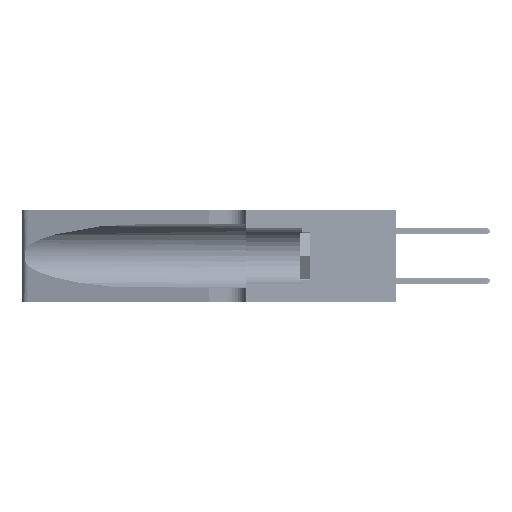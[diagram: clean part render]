
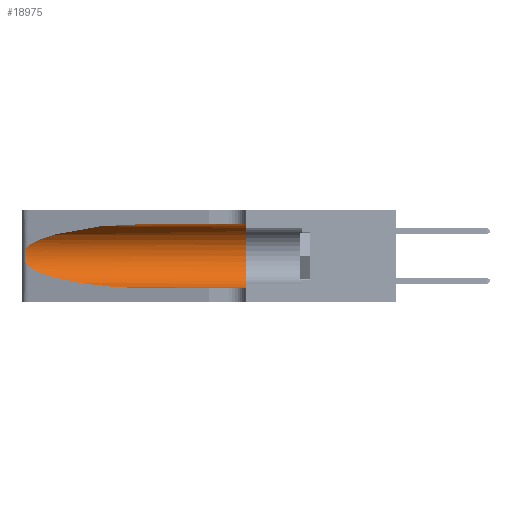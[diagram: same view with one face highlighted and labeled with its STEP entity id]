
A CAD part, left-side view. The second image highlights one B-rep face of the part: STEP entity #18975.
In plain terms, the highlighted cylindrical face has radius 3.308 mm (diameter 6.617 mm), a partial arc.
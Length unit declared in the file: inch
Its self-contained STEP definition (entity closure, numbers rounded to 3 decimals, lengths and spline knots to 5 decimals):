
#648 = EDGE_CURVE ( 'NONE', #43792, #8426, #23470, .T. ) ;
#1155 = CARTESIAN_POINT ( 'NONE',  ( 0.25487, 1.22718, 0.14631 ) ) ;
#2716 = CARTESIAN_POINT ( 'NONE',  ( 0.1305, 1.61858, 0.31525 ) ) ;
#3022 = DIRECTION ( 'NONE',  ( 0., 0., 1. ) ) ;
#4102 = CARTESIAN_POINT ( 'NONE',  ( 0.1305, 1.61858, 0.185 ) ) ;
#4693 = ORIENTED_EDGE ( 'NONE', *, *, #30047, .T. ) ;
#5092 = CARTESIAN_POINT ( 'NONE',  ( 0.25487, 1.22718, 0.14631 ) ) ;
#5726 = CARTESIAN_POINT ( 'NONE',  ( 0.26018, 1.23835, 0.19895 ) ) ;
#5967 = CIRCLE ( 'NONE', #16282, 0.13025 ) ;
#8426 = VERTEX_POINT ( 'NONE', #18879 ) ;
#8588 = CARTESIAN_POINT ( 'NONE',  ( 0.25487, 1.22718, 0.14631 ) ) ;
#9686 = CYLINDRICAL_SURFACE ( 'NONE', #45352, 0.13025 ) ;
#9708 = CARTESIAN_POINT ( 'NONE',  ( 0.1305, 0.72297, 0.31525 ) ) ;
#12324 = CARTESIAN_POINT ( 'NONE',  ( 0.1305, 0.35, 0.31525 ) ) ;
#12481 = CARTESIAN_POINT ( 'NONE',  ( 0.18966, 0.96281, 0.05475 ) ) ;
#12839 = CARTESIAN_POINT ( 'NONE',  ( 0.25639, 1.23184, 0.21858 ) ) ;
#12999 = CARTESIAN_POINT ( 'NONE',  ( 0.26017, 1.23833, 0.17102 ) ) ;
#13162 = CARTESIAN_POINT ( 'NONE',  ( 0.26075, 1.23896, 0.178 ) ) ;
#13328 = CARTESIAN_POINT ( 'NONE',  ( 0.25487, 1.22718, 0.22369 ) ) ;
#14504 = B_SPLINE_CURVE_WITH_KNOTS ( 'NONE', 3,
 ( #13328, #24491, #12839, #16703, #28889, #5726, #36243, #13162, #12999, #20458, #28718, #20939, #39790, #1155 ),
 .UNSPECIFIED., .F., .F.,
 ( 4, 2, 2, 2, 2, 2, 4 ),
 ( 0., 0.00027, 0.00053, 0.00107, 0.0016, 0.00187, 0.00214 ),
 .UNSPECIFIED. ) ;
#16282 = AXIS2_PLACEMENT_3D ( 'NONE', #44521, #41475, #3022 ) ;
#16703 = CARTESIAN_POINT ( 'NONE',  ( 0.25787, 1.23484, 0.2124 ) ) ;
#17725 = EDGE_CURVE ( 'NONE', #46839, #27034, #32550, .T. ) ;
#18879 = CARTESIAN_POINT ( 'NONE',  ( 0.25487, 1.22718, 0.22369 ) ) ;
#18975 = ADVANCED_FACE ( 'NONE', ( #29624 ), #9686, .F. ) ;
#19201 = CARTESIAN_POINT ( 'NONE',  ( 0.1305, 0.72297, 0.31525 ) ) ;
#20458 = CARTESIAN_POINT ( 'NONE',  ( 0.25856, 1.23593, 0.16098 ) ) ;
#20939 = CARTESIAN_POINT ( 'NONE',  ( 0.25639, 1.23186, 0.15144 ) ) ;
#23193 = ORIENTED_EDGE ( 'NONE', *, *, #17725, .T. ) ;
#23470 =( BOUNDED_CURVE ( )  B_SPLINE_CURVE ( 3, ( #9708, #32770, #43178, #42787 ),
 .UNSPECIFIED., .F., .T. ) 
 B_SPLINE_CURVE_WITH_KNOTS ( ( 4, 4 ),
 ( 1.5708, 2.84003 ),
 .UNSPECIFIED. ) 
 CURVE ( )  GEOMETRIC_REPRESENTATION_ITEM ( )  RATIONAL_B_SPLINE_CURVE ( ( 1., 0.87, 0.87, 1. ) ) 
 REPRESENTATION_ITEM ( '' )  );
#23532 = DIRECTION ( 'NONE',  ( 0., 0., -1. ) ) ;
#24491 = CARTESIAN_POINT ( 'NONE',  ( 0.25555, 1.22994, 0.2215 ) ) ;
#25403 = ORIENTED_EDGE ( 'NONE', *, *, #35514, .F. ) ;
#26732 = DIRECTION ( 'NONE',  ( 0., -1., 0. ) ) ;
#27034 = VERTEX_POINT ( 'NONE', #44806 ) ;
#28718 = CARTESIAN_POINT ( 'NONE',  ( 0.25789, 1.23486, 0.15765 ) ) ;
#28889 = CARTESIAN_POINT ( 'NONE',  ( 0.25854, 1.2359, 0.20912 ) ) ;
#29624 = FACE_OUTER_BOUND ( 'NONE', #37209, .T. ) ;
#30047 = EDGE_CURVE ( 'NONE', #8426, #46839, #14504, .T. ) ;
#30179 = ORIENTED_EDGE ( 'NONE', *, *, #45121, .T. ) ;
#30510 = VECTOR ( 'NONE', #34734, 39.37008 ) ;
#32107 = CARTESIAN_POINT ( 'NONE',  ( 0.1305, 0.35, 0.05475 ) ) ;
#32550 =( BOUNDED_CURVE ( )  B_SPLINE_CURVE ( 3, ( #8588, #35727, #12481, #39597 ),
 .UNSPECIFIED., .F., .F. ) 
 B_SPLINE_CURVE_WITH_KNOTS ( ( 4, 4 ),
 ( 3.44316, 4.71239 ),
 .UNSPECIFIED. ) 
 CURVE ( )  GEOMETRIC_REPRESENTATION_ITEM ( )  RATIONAL_B_SPLINE_CURVE ( ( 1., 0.87, 0.87, 1. ) ) 
 REPRESENTATION_ITEM ( '' )  );
#32770 = CARTESIAN_POINT ( 'NONE',  ( 0.18966, 0.96281, 0.31525 ) ) ;
#33622 = EDGE_CURVE ( 'NONE', #43792, #45391, #43038, .T. ) ;
#34734 = DIRECTION ( 'NONE',  ( 0., -1., 0. ) ) ;
#35514 = EDGE_CURVE ( 'NONE', #45391, #47389, #5967, .T. ) ;
#35727 = CARTESIAN_POINT ( 'NONE',  ( 0.2373, 1.15595, 0.08982 ) ) ;
#36243 = CARTESIAN_POINT ( 'NONE',  ( 0.26075, 1.23896, 0.19203 ) ) ;
#37209 = EDGE_LOOP ( 'NONE', ( #43129, #4693, #23193, #30179, #25403, #38467 ) ) ;
#38467 = ORIENTED_EDGE ( 'NONE', *, *, #33622, .F. ) ;
#39502 = DIRECTION ( 'NONE',  ( 0., -1., 0. ) ) ;
#39597 = CARTESIAN_POINT ( 'NONE',  ( 0.1305, 0.72297, 0.05475 ) ) ;
#39790 = CARTESIAN_POINT ( 'NONE',  ( 0.25555, 1.22993, 0.14849 ) ) ;
#40962 = CARTESIAN_POINT ( 'NONE',  ( 0.1305, 1.61858, 0.05475 ) ) ;
#41188 = VECTOR ( 'NONE', #26732, 39.37008 ) ;
#41475 = DIRECTION ( 'NONE',  ( 0., 1., 0. ) ) ;
#42787 = CARTESIAN_POINT ( 'NONE',  ( 0.25487, 1.22718, 0.22369 ) ) ;
#43038 = LINE ( 'NONE', #2716, #41188 ) ;
#43129 = ORIENTED_EDGE ( 'NONE', *, *, #648, .T. ) ;
#43178 = CARTESIAN_POINT ( 'NONE',  ( 0.2373, 1.15595, 0.28018 ) ) ;
#43792 = VERTEX_POINT ( 'NONE', #19201 ) ;
#44521 = CARTESIAN_POINT ( 'NONE',  ( 0.1305, 0.35, 0.185 ) ) ;
#44806 = CARTESIAN_POINT ( 'NONE',  ( 0.1305, 0.72297, 0.05475 ) ) ;
#45121 = EDGE_CURVE ( 'NONE', #27034, #47389, #48679, .T. ) ;
#45352 = AXIS2_PLACEMENT_3D ( 'NONE', #4102, #39502, #23532 ) ;
#45391 = VERTEX_POINT ( 'NONE', #12324 ) ;
#46839 = VERTEX_POINT ( 'NONE', #5092 ) ;
#47389 = VERTEX_POINT ( 'NONE', #32107 ) ;
#48679 = LINE ( 'NONE', #40962, #30510 ) ;
